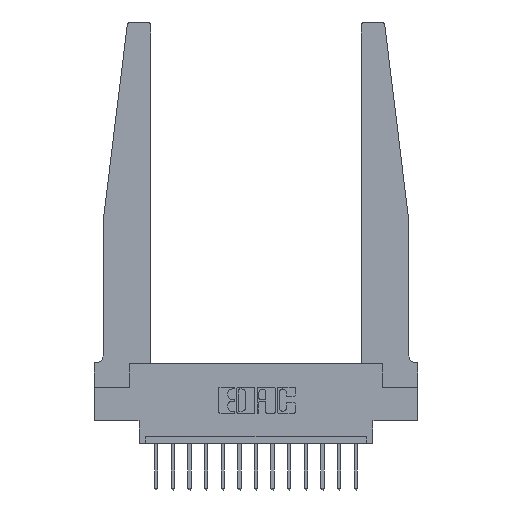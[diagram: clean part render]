
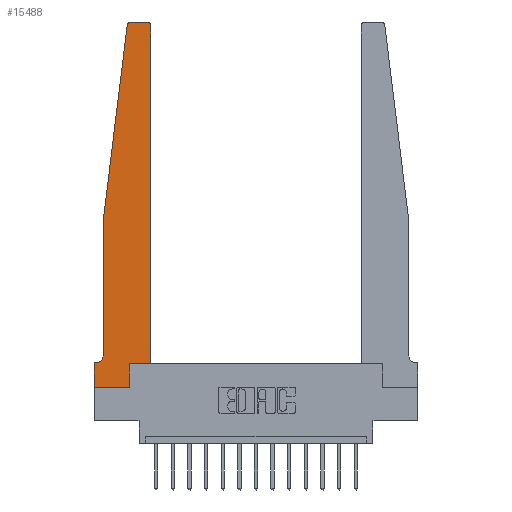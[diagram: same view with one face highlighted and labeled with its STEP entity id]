
A CAD part, top view. The second image highlights one B-rep face of the part: STEP entity #15488.
In plain terms, the highlighted planar face has unit normal (0, 0, 1).
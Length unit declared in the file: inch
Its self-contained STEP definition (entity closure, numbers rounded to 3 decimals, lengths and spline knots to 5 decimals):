
#124 = CARTESIAN_POINT ( 'NONE',  ( 0.425, 2.72, 0.37 ) ) ;
#207 = CARTESIAN_POINT ( 'NONE',  ( 0., 0., 0.37 ) ) ;
#218 = DIRECTION ( 'NONE',  ( 0., -1., 0. ) ) ;
#348 = AXIS2_PLACEMENT_3D ( 'NONE', #14160, #15333, #8852 ) ;
#538 = VERTEX_POINT ( 'NONE', #207 ) ;
#658 = VECTOR ( 'NONE', #218, 39.37008 ) ;
#795 = VERTEX_POINT ( 'NONE', #11673 ) ;
#835 = ORIENTED_EDGE ( 'NONE', *, *, #7499, .T. ) ;
#1014 = ORIENTED_EDGE ( 'NONE', *, *, #1086, .T. ) ;
#1086 = EDGE_CURVE ( 'NONE', #6448, #16430, #14835, .T. ) ;
#1121 = VERTEX_POINT ( 'NONE', #15212 ) ;
#1701 = CARTESIAN_POINT ( 'NONE',  ( 0.395, 2.72, 0.37 ) ) ;
#2131 = CARTESIAN_POINT ( 'NONE',  ( 0.065, 1.25, 0.37 ) ) ;
#2146 = VERTEX_POINT ( 'NONE', #3070 ) ;
#2305 = CARTESIAN_POINT ( 'NONE',  ( 0.065, 0.2375, 0.37 ) ) ;
#2505 = CARTESIAN_POINT ( 'NONE',  ( 0.24675, 2.72367, 0.37 ) ) ;
#2531 = EDGE_CURVE ( 'NONE', #795, #6448, #10878, .T. ) ;
#2628 = LINE ( 'NONE', #8641, #15466 ) ;
#3070 = CARTESIAN_POINT ( 'NONE',  ( 0.2605, 0., 0.37 ) ) ;
#3283 = LINE ( 'NONE', #4919, #13307 ) ;
#3309 = VERTEX_POINT ( 'NONE', #13279 ) ;
#3696 = CARTESIAN_POINT ( 'NONE',  ( 0., 0.1875, 0.37 ) ) ;
#3917 = CARTESIAN_POINT ( 'NONE',  ( 0., 0., 0.37 ) ) ;
#4131 = EDGE_CURVE ( 'NONE', #8225, #15237, #2628, .T. ) ;
#4296 = CARTESIAN_POINT ( 'NONE',  ( 0.27653, 2.75, 0.37 ) ) ;
#4450 = AXIS2_PLACEMENT_3D ( 'NONE', #1701, #9735, #10872 ) ;
#4679 = AXIS2_PLACEMENT_3D ( 'NONE', #7276, #7733, #16861 ) ;
#4919 = CARTESIAN_POINT ( 'NONE',  ( 0.065, 1.25, 0.37 ) ) ;
#4993 = ORIENTED_EDGE ( 'NONE', *, *, #8227, .T. ) ;
#5135 = VECTOR ( 'NONE', #15632, 39.37008 ) ;
#5199 = ORIENTED_EDGE ( 'NONE', *, *, #16154, .T. ) ;
#5211 = ORIENTED_EDGE ( 'NONE', *, *, #2531, .T. ) ;
#5343 = EDGE_CURVE ( 'NONE', #3309, #10244, #7880, .T. ) ;
#5563 = ORIENTED_EDGE ( 'NONE', *, *, #5343, .T. ) ;
#5667 = ORIENTED_EDGE ( 'NONE', *, *, #11036, .T. ) ;
#5759 = ORIENTED_EDGE ( 'NONE', *, *, #10425, .T. ) ;
#5786 = CIRCLE ( 'NONE', #4679, 0.05 ) ;
#5869 = VERTEX_POINT ( 'NONE', #2305 ) ;
#5949 = LINE ( 'NONE', #16702, #10691 ) ;
#6149 = ORIENTED_EDGE ( 'NONE', *, *, #14022, .T. ) ;
#6448 = VERTEX_POINT ( 'NONE', #4296 ) ;
#6463 = CARTESIAN_POINT ( 'NONE',  ( 0.25, 2.75, 0.37 ) ) ;
#6504 = DIRECTION ( 'NONE',  ( 1., 0., 0. ) ) ;
#7161 = DIRECTION ( 'NONE',  ( -0.122, -0.992, 0. ) ) ;
#7276 = CARTESIAN_POINT ( 'NONE',  ( 0.015, 0.2375, 0.37 ) ) ;
#7380 = LINE ( 'NONE', #3917, #658 ) ;
#7499 = EDGE_CURVE ( 'NONE', #5869, #8225, #5786, .T. ) ;
#7733 = DIRECTION ( 'NONE',  ( 0., 0., -1. ) ) ;
#7880 = LINE ( 'NONE', #12775, #13851 ) ;
#8225 = VERTEX_POINT ( 'NONE', #10107 ) ;
#8227 = EDGE_CURVE ( 'NONE', #16002, #5869, #3283, .T. ) ;
#8641 = CARTESIAN_POINT ( 'NONE',  ( 0.065, 0.1875, 0.37 ) ) ;
#8852 = DIRECTION ( 'NONE',  ( 1., 0., 0. ) ) ;
#8871 = CARTESIAN_POINT ( 'NONE',  ( 0., 0., 0.37 ) ) ;
#9522 = VECTOR ( 'NONE', #16244, 39.37008 ) ;
#9735 = DIRECTION ( 'NONE',  ( 0., 0., 1. ) ) ;
#9830 = DIRECTION ( 'NONE',  ( -1., 0., 0. ) ) ;
#10107 = CARTESIAN_POINT ( 'NONE',  ( 0.015, 0.1875, 0.37 ) ) ;
#10171 = DIRECTION ( 'NONE',  ( 0., -1., 0. ) ) ;
#10244 = VERTEX_POINT ( 'NONE', #124 ) ;
#10274 = DIRECTION ( 'NONE',  ( 1., 0., 0. ) ) ;
#10319 = CARTESIAN_POINT ( 'NONE',  ( 0., 0.1875, 0.37 ) ) ;
#10425 = EDGE_CURVE ( 'NONE', #2146, #1121, #12224, .T. ) ;
#10691 = VECTOR ( 'NONE', #6504, 39.37008 ) ;
#10872 = DIRECTION ( 'NONE',  ( 1., 0., 0. ) ) ;
#10878 = LINE ( 'NONE', #6463, #5135 ) ;
#11036 = EDGE_CURVE ( 'NONE', #10244, #795, #14634, .T. ) ;
#11340 = CARTESIAN_POINT ( 'NONE',  ( 0.065, 1.25, 0.37 ) ) ;
#11544 = PLANE ( 'NONE',  #15911 ) ;
#11673 = CARTESIAN_POINT ( 'NONE',  ( 0.395, 2.75, 0.37 ) ) ;
#11973 = EDGE_LOOP ( 'NONE', ( #5211, #1014, #13571, #4993, #835, #12234, #6149, #5199, #5759, #13240, #5563, #5667 ) ) ;
#12101 = VECTOR ( 'NONE', #13628, 39.37008 ) ;
#12224 = LINE ( 'NONE', #14897, #9522 ) ;
#12234 = ORIENTED_EDGE ( 'NONE', *, *, #4131, .T. ) ;
#12276 = LINE ( 'NONE', #2131, #16182 ) ;
#12775 = CARTESIAN_POINT ( 'NONE',  ( 0.425, 0.18, 0.37 ) ) ;
#13240 = ORIENTED_EDGE ( 'NONE', *, *, #13950, .T. ) ;
#13279 = CARTESIAN_POINT ( 'NONE',  ( 0.425, 0.18, 0.37 ) ) ;
#13307 = VECTOR ( 'NONE', #10171, 39.37008 ) ;
#13571 = ORIENTED_EDGE ( 'NONE', *, *, #14794, .T. ) ;
#13628 = DIRECTION ( 'NONE',  ( 1., 0., 0. ) ) ;
#13851 = VECTOR ( 'NONE', #16620, 39.37008 ) ;
#13950 = EDGE_CURVE ( 'NONE', #1121, #3309, #5949, .T. ) ;
#14022 = EDGE_CURVE ( 'NONE', #15237, #538, #7380, .T. ) ;
#14160 = CARTESIAN_POINT ( 'NONE',  ( 0.27653, 2.72, 0.37 ) ) ;
#14634 = CIRCLE ( 'NONE', #4450, 0.03 ) ;
#14794 = EDGE_CURVE ( 'NONE', #16430, #16002, #12276, .T. ) ;
#14835 = CIRCLE ( 'NONE', #348, 0.03 ) ;
#14897 = CARTESIAN_POINT ( 'NONE',  ( 0.2605, 0.18, 0.37 ) ) ;
#15212 = CARTESIAN_POINT ( 'NONE',  ( 0.2605, 0.18, 0.37 ) ) ;
#15237 = VERTEX_POINT ( 'NONE', #10319 ) ;
#15333 = DIRECTION ( 'NONE',  ( 0., 0., 1. ) ) ;
#15466 = VECTOR ( 'NONE', #9830, 39.37008 ) ;
#15488 = ADVANCED_FACE ( 'NONE', ( #16159 ), #11544, .T. ) ;
#15632 = DIRECTION ( 'NONE',  ( -1., 0., 0. ) ) ;
#15911 = AXIS2_PLACEMENT_3D ( 'NONE', #3696, #16584, #10274 ) ;
#16002 = VERTEX_POINT ( 'NONE', #11340 ) ;
#16123 = LINE ( 'NONE', #8871, #12101 ) ;
#16154 = EDGE_CURVE ( 'NONE', #538, #2146, #16123, .T. ) ;
#16159 = FACE_OUTER_BOUND ( 'NONE', #11973, .T. ) ;
#16182 = VECTOR ( 'NONE', #7161, 39.37008 ) ;
#16244 = DIRECTION ( 'NONE',  ( 0., 1., 0. ) ) ;
#16430 = VERTEX_POINT ( 'NONE', #2505 ) ;
#16584 = DIRECTION ( 'NONE',  ( 0., 0., 1. ) ) ;
#16620 = DIRECTION ( 'NONE',  ( 0., 1., 0. ) ) ;
#16702 = CARTESIAN_POINT ( 'NONE',  ( 0.425, 0.18, 0.37 ) ) ;
#16861 = DIRECTION ( 'NONE',  ( -1., 0., 0. ) ) ;
